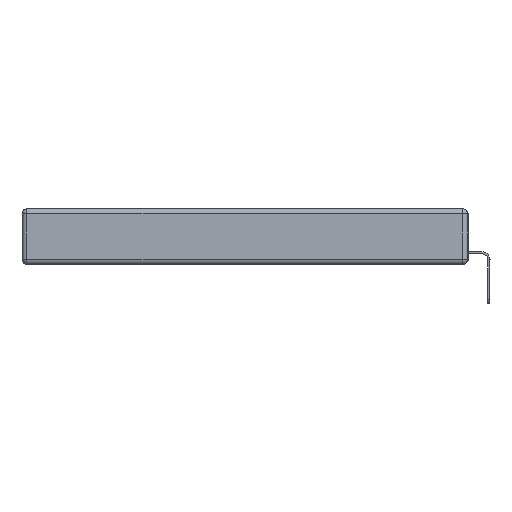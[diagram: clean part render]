
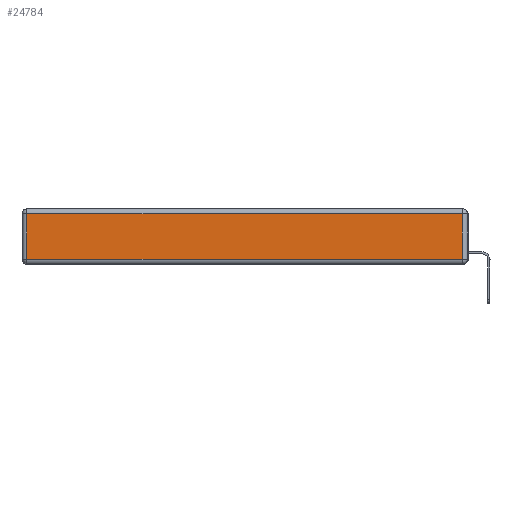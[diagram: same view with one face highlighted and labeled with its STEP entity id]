
A CAD part, left-side view. The second image highlights one B-rep face of the part: STEP entity #24784.
In plain terms, the highlighted planar face has unit normal (-1, 0, 0).
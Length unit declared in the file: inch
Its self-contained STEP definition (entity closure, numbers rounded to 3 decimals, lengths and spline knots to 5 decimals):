
#92 = CARTESIAN_POINT ( 'NONE',  ( 0., 0., -0.343 ) ) ;
#258 = CARTESIAN_POINT ( 'NONE',  ( 0., 0., -0.313 ) ) ;
#940 = VERTEX_POINT ( 'NONE', #13012 ) ;
#1469 = LINE ( 'NONE', #258, #19973 ) ;
#1846 = AXIS2_PLACEMENT_3D ( 'NONE', #92, #4389, #19428 ) ;
#2152 = ORIENTED_EDGE ( 'NONE', *, *, #5961, .T. ) ;
#2174 = VERTEX_POINT ( 'NONE', #9689 ) ;
#2458 = VECTOR ( 'NONE', #17548, 39.37008 ) ;
#2476 = CARTESIAN_POINT ( 'NONE',  ( 0., 0.03, -0.343 ) ) ;
#2586 = CARTESIAN_POINT ( 'NONE',  ( 0., 2.75, -0.03 ) ) ;
#2676 = CARTESIAN_POINT ( 'NONE',  ( 0., 2.72, -0.343 ) ) ;
#2955 = VERTEX_POINT ( 'NONE', #21936 ) ;
#4021 = LINE ( 'NONE', #2676, #16168 ) ;
#4389 = DIRECTION ( 'NONE',  ( -1., 0., 0. ) ) ;
#4549 = CARTESIAN_POINT ( 'NONE',  ( 0., 2.72, -0.03 ) ) ;
#5961 = EDGE_CURVE ( 'NONE', #940, #13064, #24734, .T. ) ;
#6161 = EDGE_LOOP ( 'NONE', ( #24743, #10461, #2152, #16901 ) ) ;
#9689 = CARTESIAN_POINT ( 'NONE',  ( 0., 0.03, -0.313 ) ) ;
#10461 = ORIENTED_EDGE ( 'NONE', *, *, #23845, .T. ) ;
#11171 = DIRECTION ( 'NONE',  ( 0., 1., 0. ) ) ;
#11843 = FACE_OUTER_BOUND ( 'NONE', #6161, .T. ) ;
#12909 = LINE ( 'NONE', #2476, #2458 ) ;
#13012 = CARTESIAN_POINT ( 'NONE',  ( 0., 0.03, -0.03 ) ) ;
#13064 = VERTEX_POINT ( 'NONE', #4549 ) ;
#13293 = VECTOR ( 'NONE', #11171, 39.37008 ) ;
#15484 = DIRECTION ( 'NONE',  ( 0., -1., 0. ) ) ;
#16168 = VECTOR ( 'NONE', #19702, 39.37008 ) ;
#16245 = EDGE_CURVE ( 'NONE', #13064, #2955, #4021, .T. ) ;
#16901 = ORIENTED_EDGE ( 'NONE', *, *, #16245, .T. ) ;
#17548 = DIRECTION ( 'NONE',  ( 0., 0., 1. ) ) ;
#19428 = DIRECTION ( 'NONE',  ( 0., 0., 1. ) ) ;
#19702 = DIRECTION ( 'NONE',  ( 0., 0., -1. ) ) ;
#19973 = VECTOR ( 'NONE', #15484, 39.37008 ) ;
#21936 = CARTESIAN_POINT ( 'NONE',  ( 0., 2.72, -0.313 ) ) ;
#23673 = PLANE ( 'NONE',  #1846 ) ;
#23845 = EDGE_CURVE ( 'NONE', #2174, #940, #12909, .T. ) ;
#23905 = EDGE_CURVE ( 'NONE', #2955, #2174, #1469, .T. ) ;
#24734 = LINE ( 'NONE', #2586, #13293 ) ;
#24743 = ORIENTED_EDGE ( 'NONE', *, *, #23905, .T. ) ;
#24784 = ADVANCED_FACE ( 'NONE', ( #11843 ), #23673, .T. ) ;
